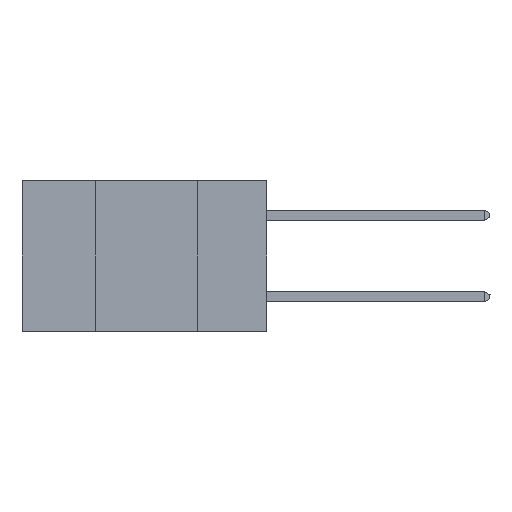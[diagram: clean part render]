
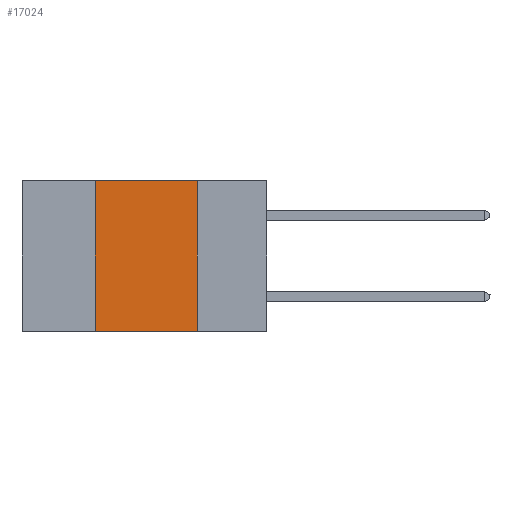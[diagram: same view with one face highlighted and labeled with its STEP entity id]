
A CAD part, left-side view. The second image highlights one B-rep face of the part: STEP entity #17024.
In plain terms, the highlighted planar face has unit normal (-1, 0, 0).
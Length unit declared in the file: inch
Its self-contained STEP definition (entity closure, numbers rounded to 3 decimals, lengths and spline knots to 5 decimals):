
#220 = AXIS2_PLACEMENT_3D ( 'NONE', #9104, #7279, #18304 ) ;
#2548 = DIRECTION ( 'NONE',  ( 0., -1., 0. ) ) ;
#2995 = VECTOR ( 'NONE', #18227, 39.37008 ) ;
#3455 = VERTEX_POINT ( 'NONE', #22122 ) ;
#3833 = ORIENTED_EDGE ( 'NONE', *, *, #22214, .F. ) ;
#4944 = EDGE_CURVE ( 'NONE', #7139, #10740, #11316, .T. ) ;
#5359 = VERTEX_POINT ( 'NONE', #16909 ) ;
#5780 = ORIENTED_EDGE ( 'NONE', *, *, #6828, .F. ) ;
#6828 = EDGE_CURVE ( 'NONE', #5359, #10740, #22524, .T. ) ;
#7139 = VERTEX_POINT ( 'NONE', #15794 ) ;
#7279 = DIRECTION ( 'NONE',  ( 1., 0., 0. ) ) ;
#8366 = LINE ( 'NONE', #12883, #2995 ) ;
#9104 = CARTESIAN_POINT ( 'NONE',  ( 0., 0.6, 0. ) ) ;
#9194 = CARTESIAN_POINT ( 'NONE',  ( 0., 0.6, 0. ) ) ;
#9916 = EDGE_CURVE ( 'NONE', #3455, #5359, #9996, .T. ) ;
#9996 = LINE ( 'NONE', #9194, #21235 ) ;
#10199 = ORIENTED_EDGE ( 'NONE', *, *, #9916, .F. ) ;
#10740 = VERTEX_POINT ( 'NONE', #11449 ) ;
#10913 = ORIENTED_EDGE ( 'NONE', *, *, #4944, .T. ) ;
#11316 = LINE ( 'NONE', #13097, #17227 ) ;
#11449 = CARTESIAN_POINT ( 'NONE',  ( 0., 0.17, -0.37 ) ) ;
#12470 = EDGE_LOOP ( 'NONE', ( #5780, #10199, #3833, #10913 ) ) ;
#12883 = CARTESIAN_POINT ( 'NONE',  ( 0., 0.42, 0. ) ) ;
#13097 = CARTESIAN_POINT ( 'NONE',  ( 0., 0.6, -0.37 ) ) ;
#15794 = CARTESIAN_POINT ( 'NONE',  ( 0., 0.42, -0.37 ) ) ;
#16909 = CARTESIAN_POINT ( 'NONE',  ( 0., 0.17, 0. ) ) ;
#17024 = ADVANCED_FACE ( 'NONE', ( #19906 ), #18068, .F. ) ;
#17227 = VECTOR ( 'NONE', #2548, 39.37008 ) ;
#18068 = PLANE ( 'NONE',  #220 ) ;
#18227 = DIRECTION ( 'NONE',  ( 0., 0., 1. ) ) ;
#18304 = DIRECTION ( 'NONE',  ( 0., 0., -1. ) ) ;
#18346 = CARTESIAN_POINT ( 'NONE',  ( 0., 0.17, 0. ) ) ;
#19906 = FACE_OUTER_BOUND ( 'NONE', #12470, .T. ) ;
#21235 = VECTOR ( 'NONE', #21863, 39.37008 ) ;
#21863 = DIRECTION ( 'NONE',  ( 0., -1., 0. ) ) ;
#21968 = VECTOR ( 'NONE', #22192, 39.37008 ) ;
#22122 = CARTESIAN_POINT ( 'NONE',  ( 0., 0.42, 0. ) ) ;
#22192 = DIRECTION ( 'NONE',  ( 0., 0., -1. ) ) ;
#22214 = EDGE_CURVE ( 'NONE', #7139, #3455, #8366, .T. ) ;
#22524 = LINE ( 'NONE', #18346, #21968 ) ;
